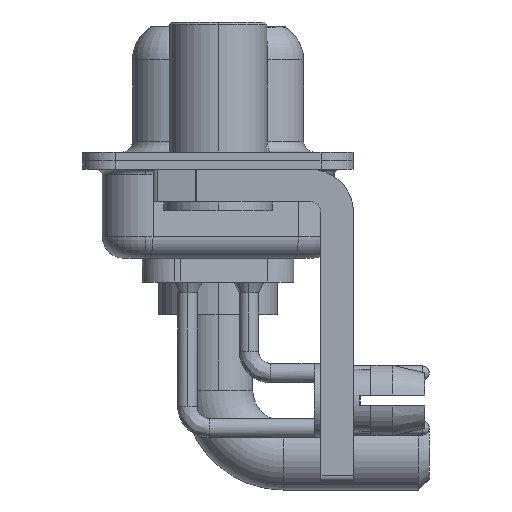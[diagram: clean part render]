
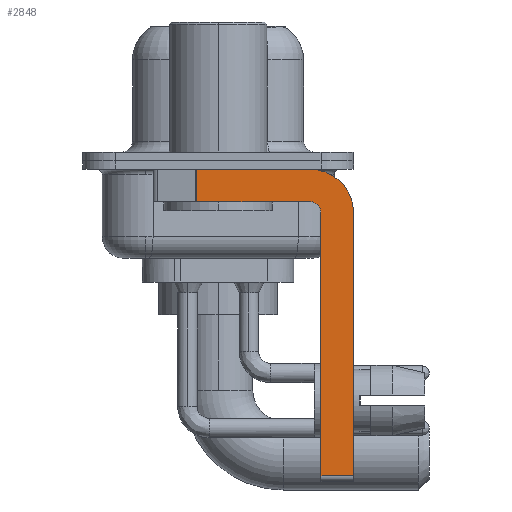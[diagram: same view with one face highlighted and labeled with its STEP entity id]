
A CAD part, left-side view. The second image highlights one B-rep face of the part: STEP entity #2848.
In plain terms, the highlighted planar face has unit normal (-1, 0, 0).
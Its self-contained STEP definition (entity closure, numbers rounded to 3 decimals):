
#21 = EDGE_CURVE ( 'NONE', #4228, #11851, #375, .T. ) ;
#375 = LINE ( 'NONE', #5239, #2362 ) ;
#381 = CARTESIAN_POINT ( 'NONE',  ( -2.9, -4.25, -0.4 ) ) ;
#727 = CARTESIAN_POINT ( 'NONE',  ( -2.9, -6.25, -14.55 ) ) ;
#1513 = EDGE_CURVE ( 'NONE', #11352, #21761, #20941, .T. ) ;
#1694 = VERTEX_POINT ( 'NONE', #5450 ) ;
#2188 = CARTESIAN_POINT ( 'NONE',  ( -2.9, -4.25, -1.9 ) ) ;
#2362 = VECTOR ( 'NONE', #9269, 1000. ) ;
#2550 = CARTESIAN_POINT ( 'NONE',  ( -2.9, -4.75, -2.4 ) ) ;
#2592 = CARTESIAN_POINT ( 'NONE',  ( -2.9, -4.25, -1.9 ) ) ;
#2615 = CARTESIAN_POINT ( 'NONE',  ( -2.9, -4.75, -14.8 ) ) ;
#2848 = ADVANCED_FACE ( 'NONE', ( #15237 ), #3336, .F. ) ;
#3336 = PLANE ( 'NONE',  #7461 ) ;
#3636 = VERTEX_POINT ( 'NONE', #2592 ) ;
#3684 = CARTESIAN_POINT ( 'NONE',  ( -2.9, 0.978, -0.4 ) ) ;
#3759 = CARTESIAN_POINT ( 'NONE',  ( -2.9, 0.978, -1.9 ) ) ;
#3917 = LINE ( 'NONE', #2188, #7643 ) ;
#4228 = VERTEX_POINT ( 'NONE', #3684 ) ;
#4346 = EDGE_CURVE ( 'NONE', #3636, #14087, #3917, .T. ) ;
#5239 = CARTESIAN_POINT ( 'NONE',  ( -2.9, 3., -0.4 ) ) ;
#5450 = CARTESIAN_POINT ( 'NONE',  ( -2.9, -6.25, -2.4 ) ) ;
#5893 = ORIENTED_EDGE ( 'NONE', *, *, #15699, .T. ) ;
#6404 = VECTOR ( 'NONE', #20316, 1000. ) ;
#6491 = VECTOR ( 'NONE', #9422, 1000. ) ;
#6578 = CARTESIAN_POINT ( 'NONE',  ( -2.9, -4.25, -2.4 ) ) ;
#7048 = DIRECTION ( 'NONE',  ( -1., 0., 0. ) ) ;
#7229 = ORIENTED_EDGE ( 'NONE', *, *, #10221, .F. ) ;
#7461 = AXIS2_PLACEMENT_3D ( 'NONE', #6578, #10383, #12007 ) ;
#7643 = VECTOR ( 'NONE', #18008, 1000. ) ;
#7663 = ORIENTED_EDGE ( 'NONE', *, *, #20508, .T. ) ;
#8034 = LINE ( 'NONE', #11383, #11489 ) ;
#8472 = CARTESIAN_POINT ( 'NONE',  ( -2.9, -4.25, -2.4 ) ) ;
#8516 = EDGE_LOOP ( 'NONE', ( #8917, #5893, #14559, #21401, #22553, #7663, #7229, #18965 ) ) ;
#8917 = ORIENTED_EDGE ( 'NONE', *, *, #21, .F. ) ;
#9269 = DIRECTION ( 'NONE',  ( 0., -1., 0. ) ) ;
#9422 = DIRECTION ( 'NONE',  ( 0., 0., -1. ) ) ;
#9896 = DIRECTION ( 'NONE',  ( 0., 0., 1. ) ) ;
#10221 = EDGE_CURVE ( 'NONE', #1694, #12962, #8034, .T. ) ;
#10338 = EDGE_CURVE ( 'NONE', #11851, #1694, #17779, .T. ) ;
#10383 = DIRECTION ( 'NONE',  ( 1., 0., 0. ) ) ;
#10830 = CARTESIAN_POINT ( 'NONE',  ( -2.9, 0.978, -1.9 ) ) ;
#11352 = VERTEX_POINT ( 'NONE', #21551 ) ;
#11383 = CARTESIAN_POINT ( 'NONE',  ( -2.9, -6.25, -2.4 ) ) ;
#11489 = VECTOR ( 'NONE', #13116, 1000. ) ;
#11851 = VERTEX_POINT ( 'NONE', #381 ) ;
#12007 = DIRECTION ( 'NONE',  ( 0., 0., -1. ) ) ;
#12156 = EDGE_CURVE ( 'NONE', #21761, #3636, #17467, .T. ) ;
#12375 = DIRECTION ( 'NONE',  ( 0., 0., 1. ) ) ;
#12962 = VERTEX_POINT ( 'NONE', #727 ) ;
#13116 = DIRECTION ( 'NONE',  ( 0., 0., -1. ) ) ;
#13989 = VECTOR ( 'NONE', #9896, 1000. ) ;
#14087 = VERTEX_POINT ( 'NONE', #10830 ) ;
#14559 = ORIENTED_EDGE ( 'NONE', *, *, #4346, .F. ) ;
#15237 = FACE_OUTER_BOUND ( 'NONE', #8516, .T. ) ;
#15504 = DIRECTION ( 'NONE',  ( 1., 0., 0. ) ) ;
#15699 = EDGE_CURVE ( 'NONE', #4228, #14087, #21431, .T. ) ;
#17467 = CIRCLE ( 'NONE', #21176, 0.5 ) ;
#17779 = CIRCLE ( 'NONE', #22574, 2. ) ;
#18008 = DIRECTION ( 'NONE',  ( 0., 1., 0. ) ) ;
#18117 = LINE ( 'NONE', #21590, #6404 ) ;
#18965 = ORIENTED_EDGE ( 'NONE', *, *, #10338, .F. ) ;
#20316 = DIRECTION ( 'NONE',  ( 0., -1., 0. ) ) ;
#20508 = EDGE_CURVE ( 'NONE', #11352, #12962, #18117, .T. ) ;
#20941 = LINE ( 'NONE', #2615, #13989 ) ;
#21176 = AXIS2_PLACEMENT_3D ( 'NONE', #21382, #7048, #12375 ) ;
#21382 = CARTESIAN_POINT ( 'NONE',  ( -2.9, -4.25, -2.4 ) ) ;
#21401 = ORIENTED_EDGE ( 'NONE', *, *, #12156, .F. ) ;
#21431 = LINE ( 'NONE', #3759, #6491 ) ;
#21551 = CARTESIAN_POINT ( 'NONE',  ( -2.9, -4.75, -14.55 ) ) ;
#21590 = CARTESIAN_POINT ( 'NONE',  ( -2.9, -4.25, -14.55 ) ) ;
#21761 = VERTEX_POINT ( 'NONE', #2550 ) ;
#22553 = ORIENTED_EDGE ( 'NONE', *, *, #1513, .F. ) ;
#22559 = DIRECTION ( 'NONE',  ( 0., 0., -1. ) ) ;
#22574 = AXIS2_PLACEMENT_3D ( 'NONE', #8472, #15504, #22559 ) ;
